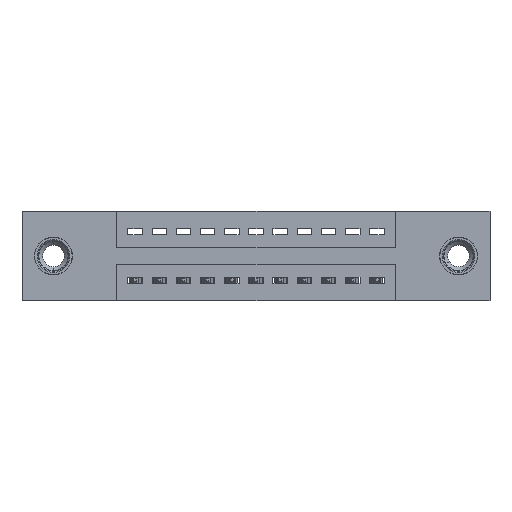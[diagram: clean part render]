
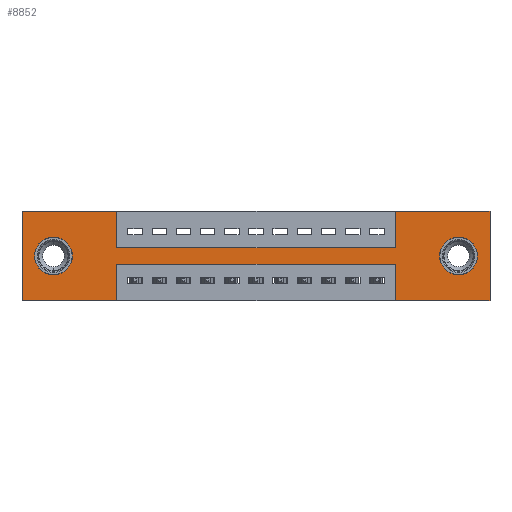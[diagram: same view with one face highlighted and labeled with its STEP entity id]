
A CAD part, front view. The second image highlights one B-rep face of the part: STEP entity #8852.
In plain terms, the highlighted planar face has unit normal (0, -1, 0).
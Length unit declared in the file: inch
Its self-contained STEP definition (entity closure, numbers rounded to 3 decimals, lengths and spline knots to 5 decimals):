
#28 = CARTESIAN_POINT ( 'NONE',  ( 1.5425, 0., -0.15 ) ) ;
#237 = CIRCLE ( 'NONE', #11007, 0.078 ) ;
#425 = CARTESIAN_POINT ( 'NONE',  ( 0.3925, 0., -0.15 ) ) ;
#473 = DIRECTION ( 'NONE',  ( -1., 0., 0. ) ) ;
#592 = VERTEX_POINT ( 'NONE', #1886 ) ;
#651 = PLANE ( 'NONE',  #11536 ) ;
#1141 = VECTOR ( 'NONE', #5324, 39.37008 ) ;
#1184 = EDGE_CURVE ( 'NONE', #7679, #12078, #13365, .T. ) ;
#1187 = EDGE_CURVE ( 'NONE', #4583, #5505, #9477, .T. ) ;
#1205 = ORIENTED_EDGE ( 'NONE', *, *, #1187, .F. ) ;
#1300 = FACE_BOUND ( 'NONE', #13059, .T. ) ;
#1546 = CARTESIAN_POINT ( 'NONE',  ( 0.3925, 0., -0.15 ) ) ;
#1740 = ORIENTED_EDGE ( 'NONE', *, *, #6438, .F. ) ;
#1884 = AXIS2_PLACEMENT_3D ( 'NONE', #9716, #7511, #2248 ) ;
#1886 = CARTESIAN_POINT ( 'NONE',  ( 0.13, 0., -0.107 ) ) ;
#1914 = VERTEX_POINT ( 'NONE', #9759 ) ;
#1923 = CARTESIAN_POINT ( 'NONE',  ( 0., 0., -0.37 ) ) ;
#2008 = DIRECTION ( 'NONE',  ( 0., 1., 0. ) ) ;
#2248 = DIRECTION ( 'NONE',  ( 0., 0., -1. ) ) ;
#2516 = DIRECTION ( 'NONE',  ( 1., 0., 0. ) ) ;
#2535 = DIRECTION ( 'NONE',  ( 1., 0., 0. ) ) ;
#2554 = CARTESIAN_POINT ( 'NONE',  ( 1.5425, 0., 0. ) ) ;
#2630 = EDGE_CURVE ( 'NONE', #5919, #11712, #10068, .T. ) ;
#2812 = VECTOR ( 'NONE', #2535, 39.37008 ) ;
#3089 = CARTESIAN_POINT ( 'NONE',  ( 0., 0., -0.37 ) ) ;
#3127 = ORIENTED_EDGE ( 'NONE', *, *, #9073, .F. ) ;
#3146 = DIRECTION ( 'NONE',  ( 0., 1., 0. ) ) ;
#3168 = EDGE_CURVE ( 'NONE', #12078, #11121, #3438, .T. ) ;
#3235 = CARTESIAN_POINT ( 'NONE',  ( 0., 0., 0. ) ) ;
#3286 = VECTOR ( 'NONE', #11098, 39.37008 ) ;
#3438 = LINE ( 'NONE', #8657, #3286 ) ;
#3595 = CARTESIAN_POINT ( 'NONE',  ( 1.935, 0., -0.37 ) ) ;
#3715 = CIRCLE ( 'NONE', #1884, 0.078 ) ;
#3735 = CARTESIAN_POINT ( 'NONE',  ( 1.5425, 0., -0.37 ) ) ;
#3752 = ORIENTED_EDGE ( 'NONE', *, *, #5470, .F. ) ;
#3804 = DIRECTION ( 'NONE',  ( -1., 0., 0. ) ) ;
#4003 = DIRECTION ( 'NONE',  ( 0., 0., -1. ) ) ;
#4124 = CARTESIAN_POINT ( 'NONE',  ( 0., 0., -0.37 ) ) ;
#4247 = ORIENTED_EDGE ( 'NONE', *, *, #13386, .F. ) ;
#4281 = LINE ( 'NONE', #7915, #12992 ) ;
#4299 = CARTESIAN_POINT ( 'NONE',  ( 1.935, 0., 0. ) ) ;
#4303 = DIRECTION ( 'NONE',  ( 1., 0., 0. ) ) ;
#4583 = VERTEX_POINT ( 'NONE', #9197 ) ;
#4777 = CARTESIAN_POINT ( 'NONE',  ( 0., 0., -0.37 ) ) ;
#4794 = EDGE_CURVE ( 'NONE', #12981, #10260, #3715, .T. ) ;
#4857 = ORIENTED_EDGE ( 'NONE', *, *, #1184, .F. ) ;
#4931 = DIRECTION ( 'NONE',  ( 0., 0., 1. ) ) ;
#5280 = CARTESIAN_POINT ( 'NONE',  ( 0.3925, 0., 0. ) ) ;
#5315 = CARTESIAN_POINT ( 'NONE',  ( 1.5425, 0., 0. ) ) ;
#5324 = DIRECTION ( 'NONE',  ( 0., 0., -1. ) ) ;
#5412 = ORIENTED_EDGE ( 'NONE', *, *, #3168, .F. ) ;
#5470 = EDGE_CURVE ( 'NONE', #1914, #6475, #13576, .T. ) ;
#5505 = VERTEX_POINT ( 'NONE', #8758 ) ;
#5607 = CARTESIAN_POINT ( 'NONE',  ( 0.3925, 0., 0. ) ) ;
#5647 = ORIENTED_EDGE ( 'NONE', *, *, #2630, .F. ) ;
#5715 = DIRECTION ( 'NONE',  ( 0., 0., -1. ) ) ;
#5889 = DIRECTION ( 'NONE',  ( 0., 0., 1. ) ) ;
#5919 = VERTEX_POINT ( 'NONE', #3735 ) ;
#6186 = CARTESIAN_POINT ( 'NONE',  ( 1.805, 0., -0.185 ) ) ;
#6335 = EDGE_CURVE ( 'NONE', #10260, #12981, #8936, .T. ) ;
#6402 = CARTESIAN_POINT ( 'NONE',  ( 0.13, 0., -0.185 ) ) ;
#6438 = EDGE_CURVE ( 'NONE', #5505, #7161, #10103, .T. ) ;
#6475 = VERTEX_POINT ( 'NONE', #5607 ) ;
#6626 = VECTOR ( 'NONE', #5715, 39.37008 ) ;
#6772 = EDGE_CURVE ( 'NONE', #9529, #592, #8755, .T. ) ;
#6851 = CARTESIAN_POINT ( 'NONE',  ( 1.5425, 0., -0.37 ) ) ;
#7014 = AXIS2_PLACEMENT_3D ( 'NONE', #6402, #3146, #9484 ) ;
#7058 = VECTOR ( 'NONE', #4931, 39.37008 ) ;
#7161 = VERTEX_POINT ( 'NONE', #4124 ) ;
#7264 = VERTEX_POINT ( 'NONE', #28 ) ;
#7511 = DIRECTION ( 'NONE',  ( 0., 1., 0. ) ) ;
#7529 = EDGE_CURVE ( 'NONE', #9480, #7264, #9898, .T. ) ;
#7679 = VERTEX_POINT ( 'NONE', #5315 ) ;
#7915 = CARTESIAN_POINT ( 'NONE',  ( 0.3925, 0., -0.22 ) ) ;
#8026 = DIRECTION ( 'NONE',  ( 0., -1., 0. ) ) ;
#8047 = CARTESIAN_POINT ( 'NONE',  ( 1.5425, 0., -0.22 ) ) ;
#8205 = VECTOR ( 'NONE', #473, 39.37008 ) ;
#8265 = EDGE_CURVE ( 'NONE', #7161, #1914, #11505, .T. ) ;
#8333 = ORIENTED_EDGE ( 'NONE', *, *, #9230, .F. ) ;
#8377 = DIRECTION ( 'NONE',  ( -1., 0., 0. ) ) ;
#8438 = EDGE_CURVE ( 'NONE', #6475, #9480, #9048, .T. ) ;
#8562 = CARTESIAN_POINT ( 'NONE',  ( 1.805, 0., -0.263 ) ) ;
#8657 = CARTESIAN_POINT ( 'NONE',  ( 1.935, 0., 0. ) ) ;
#8755 = CIRCLE ( 'NONE', #7014, 0.078 ) ;
#8758 = CARTESIAN_POINT ( 'NONE',  ( 0.3925, 0., -0.37 ) ) ;
#8806 = VECTOR ( 'NONE', #4303, 39.37008 ) ;
#8823 = VECTOR ( 'NONE', #5889, 39.37008 ) ;
#8826 = ORIENTED_EDGE ( 'NONE', *, *, #8265, .F. ) ;
#8852 = ADVANCED_FACE ( 'NONE', ( #12511, #1300, #11337 ), #651, .T. ) ;
#8899 = CARTESIAN_POINT ( 'NONE',  ( 0.13, 0., -0.185 ) ) ;
#8936 = CIRCLE ( 'NONE', #12032, 0.078 ) ;
#8959 = ORIENTED_EDGE ( 'NONE', *, *, #7529, .F. ) ;
#9048 = LINE ( 'NONE', #5280, #1141 ) ;
#9073 = EDGE_CURVE ( 'NONE', #11121, #5919, #12840, .T. ) ;
#9106 = CARTESIAN_POINT ( 'NONE',  ( 1.805, 0., -0.107 ) ) ;
#9143 = DIRECTION ( 'NONE',  ( 0., 0., 1. ) ) ;
#9197 = CARTESIAN_POINT ( 'NONE',  ( 0.3925, 0., -0.22 ) ) ;
#9230 = EDGE_CURVE ( 'NONE', #11712, #4583, #4281, .T. ) ;
#9477 = LINE ( 'NONE', #9862, #6626 ) ;
#9480 = VERTEX_POINT ( 'NONE', #425 ) ;
#9484 = DIRECTION ( 'NONE',  ( 0., 0., 1. ) ) ;
#9529 = VERTEX_POINT ( 'NONE', #9567 ) ;
#9567 = CARTESIAN_POINT ( 'NONE',  ( 0.13, 0., -0.263 ) ) ;
#9648 = ORIENTED_EDGE ( 'NONE', *, *, #10356, .T. ) ;
#9716 = CARTESIAN_POINT ( 'NONE',  ( 1.805, 0., -0.185 ) ) ;
#9759 = CARTESIAN_POINT ( 'NONE',  ( 0., 0., 0. ) ) ;
#9862 = CARTESIAN_POINT ( 'NONE',  ( 0.3925, 0., -0.37 ) ) ;
#9883 = DIRECTION ( 'NONE',  ( 0., 0., 1. ) ) ;
#9898 = LINE ( 'NONE', #1546, #2812 ) ;
#9974 = DIRECTION ( 'NONE',  ( 0., 1., 0. ) ) ;
#10068 = LINE ( 'NONE', #6851, #7058 ) ;
#10103 = LINE ( 'NONE', #3089, #11217 ) ;
#10162 = LINE ( 'NONE', #2554, #8823 ) ;
#10260 = VERTEX_POINT ( 'NONE', #8562 ) ;
#10356 = EDGE_CURVE ( 'NONE', #592, #9529, #237, .T. ) ;
#10685 = ORIENTED_EDGE ( 'NONE', *, *, #6335, .T. ) ;
#11007 = AXIS2_PLACEMENT_3D ( 'NONE', #8899, #9974, #9883 ) ;
#11098 = DIRECTION ( 'NONE',  ( 0., 0., -1. ) ) ;
#11103 = CARTESIAN_POINT ( 'NONE',  ( 0., 0., 0. ) ) ;
#11109 = ORIENTED_EDGE ( 'NONE', *, *, #6772, .T. ) ;
#11121 = VERTEX_POINT ( 'NONE', #3595 ) ;
#11217 = VECTOR ( 'NONE', #8377, 39.37008 ) ;
#11337 = FACE_OUTER_BOUND ( 'NONE', #12038, .T. ) ;
#11412 = ORIENTED_EDGE ( 'NONE', *, *, #4794, .T. ) ;
#11505 = LINE ( 'NONE', #11103, #13301 ) ;
#11536 = AXIS2_PLACEMENT_3D ( 'NONE', #1923, #8026, #4003 ) ;
#11712 = VERTEX_POINT ( 'NONE', #8047 ) ;
#12032 = AXIS2_PLACEMENT_3D ( 'NONE', #6186, #2008, #12540 ) ;
#12038 = EDGE_LOOP ( 'NONE', ( #1205, #8333, #5647, #3127, #5412, #4857, #4247, #8959, #12723, #3752, #8826, #1740 ) ) ;
#12078 = VERTEX_POINT ( 'NONE', #4299 ) ;
#12232 = VECTOR ( 'NONE', #2516, 39.37008 ) ;
#12511 = FACE_BOUND ( 'NONE', #12622, .T. ) ;
#12540 = DIRECTION ( 'NONE',  ( 0., 0., -1. ) ) ;
#12622 = EDGE_LOOP ( 'NONE', ( #11412, #10685 ) ) ;
#12723 = ORIENTED_EDGE ( 'NONE', *, *, #8438, .F. ) ;
#12840 = LINE ( 'NONE', #4777, #8205 ) ;
#12887 = CARTESIAN_POINT ( 'NONE',  ( 0., 0., 0. ) ) ;
#12981 = VERTEX_POINT ( 'NONE', #9106 ) ;
#12992 = VECTOR ( 'NONE', #3804, 39.37008 ) ;
#13059 = EDGE_LOOP ( 'NONE', ( #9648, #11109 ) ) ;
#13301 = VECTOR ( 'NONE', #9143, 39.37008 ) ;
#13365 = LINE ( 'NONE', #12887, #12232 ) ;
#13386 = EDGE_CURVE ( 'NONE', #7264, #7679, #10162, .T. ) ;
#13576 = LINE ( 'NONE', #3235, #8806 ) ;
